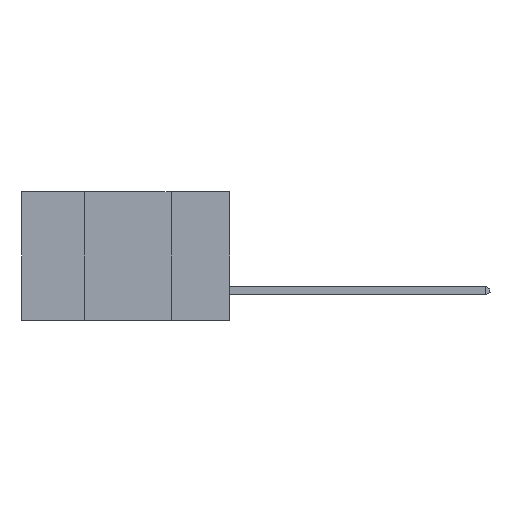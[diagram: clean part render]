
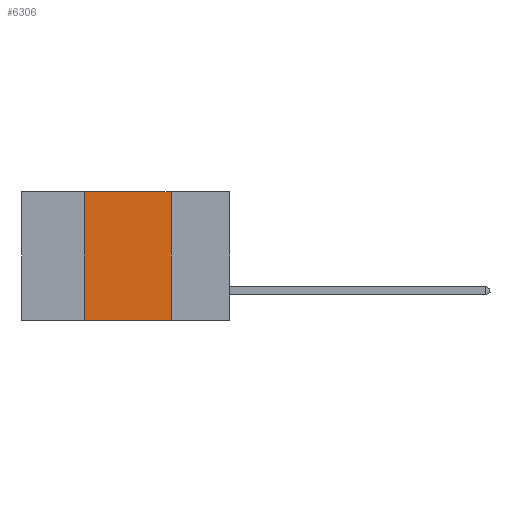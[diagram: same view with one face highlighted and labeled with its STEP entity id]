
A CAD part, left-side view. The second image highlights one B-rep face of the part: STEP entity #6306.
In plain terms, the highlighted planar face has unit normal (-1, 0, 0).
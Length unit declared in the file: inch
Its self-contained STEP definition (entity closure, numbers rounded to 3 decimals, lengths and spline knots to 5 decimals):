
#317 = DIRECTION ( 'NONE',  ( 1., 0., 0. ) ) ;
#1350 = CARTESIAN_POINT ( 'NONE',  ( 0., 0.42, -0.37 ) ) ;
#1494 = CARTESIAN_POINT ( 'NONE',  ( 0., 0.42, 0. ) ) ;
#1778 = DIRECTION ( 'NONE',  ( 0., -1., 0. ) ) ;
#1935 = VERTEX_POINT ( 'NONE', #22893 ) ;
#2280 = DIRECTION ( 'NONE',  ( 0., 0., -1. ) ) ;
#2474 = DIRECTION ( 'NONE',  ( 0., 0., -1. ) ) ;
#4422 = FACE_OUTER_BOUND ( 'NONE', #6671, .T. ) ;
#4802 = VECTOR ( 'NONE', #2280, 39.37008 ) ;
#5057 = ORIENTED_EDGE ( 'NONE', *, *, #23173, .F. ) ;
#5538 = DIRECTION ( 'NONE',  ( 0., -1., 0. ) ) ;
#5562 = CARTESIAN_POINT ( 'NONE',  ( 0., 0.42, 0. ) ) ;
#6306 = ADVANCED_FACE ( 'NONE', ( #4422 ), #8189, .F. ) ;
#6671 = EDGE_LOOP ( 'NONE', ( #19864, #5057, #10495, #15473 ) ) ;
#7097 = AXIS2_PLACEMENT_3D ( 'NONE', #25612, #317, #2474 ) ;
#8189 = PLANE ( 'NONE',  #7097 ) ;
#9261 = VECTOR ( 'NONE', #16362, 39.37008 ) ;
#9681 = EDGE_CURVE ( 'NONE', #24397, #1935, #25785, .T. ) ;
#10495 = ORIENTED_EDGE ( 'NONE', *, *, #15315, .F. ) ;
#10670 = VECTOR ( 'NONE', #1778, 39.37008 ) ;
#10904 = LINE ( 'NONE', #5562, #9261 ) ;
#10972 = EDGE_CURVE ( 'NONE', #15880, #1935, #22490, .T. ) ;
#12236 = CARTESIAN_POINT ( 'NONE',  ( 0., 0.6, 0. ) ) ;
#15315 = EDGE_CURVE ( 'NONE', #24397, #21858, #10904, .T. ) ;
#15473 = ORIENTED_EDGE ( 'NONE', *, *, #9681, .T. ) ;
#15880 = VERTEX_POINT ( 'NONE', #26528 ) ;
#16362 = DIRECTION ( 'NONE',  ( 0., 0., 1. ) ) ;
#19864 = ORIENTED_EDGE ( 'NONE', *, *, #10972, .F. ) ;
#21055 = CARTESIAN_POINT ( 'NONE',  ( 0., 0.17, 0. ) ) ;
#21858 = VERTEX_POINT ( 'NONE', #1494 ) ;
#22490 = LINE ( 'NONE', #21055, #4802 ) ;
#22893 = CARTESIAN_POINT ( 'NONE',  ( 0., 0.17, -0.37 ) ) ;
#23173 = EDGE_CURVE ( 'NONE', #21858, #15880, #24388, .T. ) ;
#24388 = LINE ( 'NONE', #12236, #10670 ) ;
#24397 = VERTEX_POINT ( 'NONE', #1350 ) ;
#25612 = CARTESIAN_POINT ( 'NONE',  ( 0., 0.6, 0. ) ) ;
#25785 = LINE ( 'NONE', #25998, #26757 ) ;
#25998 = CARTESIAN_POINT ( 'NONE',  ( 0., 0.6, -0.37 ) ) ;
#26528 = CARTESIAN_POINT ( 'NONE',  ( 0., 0.17, 0. ) ) ;
#26757 = VECTOR ( 'NONE', #5538, 39.37008 ) ;
